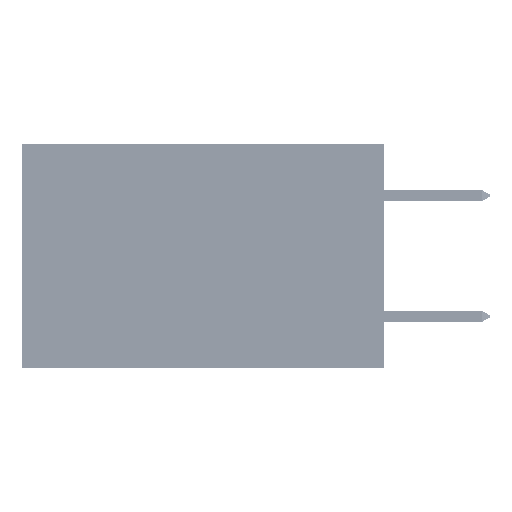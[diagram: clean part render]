
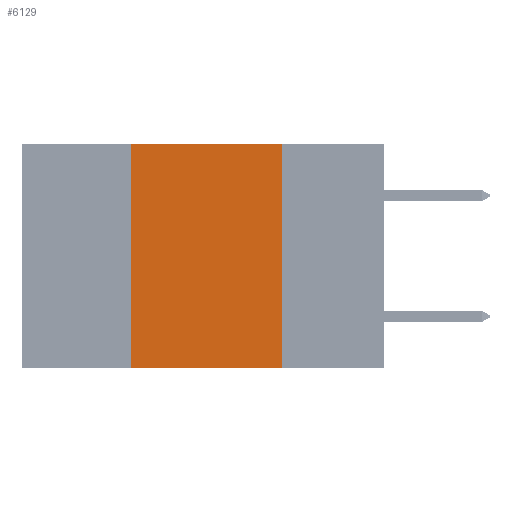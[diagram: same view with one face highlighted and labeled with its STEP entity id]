
A CAD part, left-side view. The second image highlights one B-rep face of the part: STEP entity #6129.
In plain terms, the highlighted planar face has unit normal (-1, 0, 0).
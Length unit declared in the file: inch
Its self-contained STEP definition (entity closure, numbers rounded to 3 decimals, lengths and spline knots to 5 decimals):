
#856 = EDGE_CURVE ( 'NONE', #33650, #27163, #22247, .T. ) ;
#1186 = VECTOR ( 'NONE', #45762, 39.37008 ) ;
#2209 = EDGE_CURVE ( 'NONE', #26394, #33452, #11056, .T. ) ;
#2856 = CARTESIAN_POINT ( 'NONE',  ( 0., 0.17, 0. ) ) ;
#3942 = EDGE_CURVE ( 'NONE', #26394, #33650, #14056, .T. ) ;
#6129 = ADVANCED_FACE ( 'NONE', ( #16277 ), #30497, .F. ) ;
#7517 = CARTESIAN_POINT ( 'NONE',  ( 0., 0.42, 0. ) ) ;
#9298 = DIRECTION ( 'NONE',  ( 0., 0., -1. ) ) ;
#10473 = DIRECTION ( 'NONE',  ( 0., 0., -1. ) ) ;
#10934 = CARTESIAN_POINT ( 'NONE',  ( 0., 0.42, -0.37 ) ) ;
#11056 = LINE ( 'NONE', #17357, #1186 ) ;
#11306 = ORIENTED_EDGE ( 'NONE', *, *, #2209, .T. ) ;
#12801 = DIRECTION ( 'NONE',  ( 1., 0., 0. ) ) ;
#13345 = CARTESIAN_POINT ( 'NONE',  ( 0., 0.17, -0.37 ) ) ;
#13594 = AXIS2_PLACEMENT_3D ( 'NONE', #44694, #12801, #9298 ) ;
#14056 = LINE ( 'NONE', #7517, #21716 ) ;
#15438 = VECTOR ( 'NONE', #33174, 39.37008 ) ;
#16277 = FACE_OUTER_BOUND ( 'NONE', #37872, .T. ) ;
#17357 = CARTESIAN_POINT ( 'NONE',  ( 0., 0.6, -0.37 ) ) ;
#19200 = CARTESIAN_POINT ( 'NONE',  ( 0., 0.6, 0. ) ) ;
#21716 = VECTOR ( 'NONE', #28941, 39.37008 ) ;
#22247 = LINE ( 'NONE', #19200, #15438 ) ;
#22979 = ORIENTED_EDGE ( 'NONE', *, *, #31067, .F. ) ;
#23288 = CARTESIAN_POINT ( 'NONE',  ( 0., 0.42, 0. ) ) ;
#26394 = VERTEX_POINT ( 'NONE', #10934 ) ;
#27163 = VERTEX_POINT ( 'NONE', #2856 ) ;
#27729 = VECTOR ( 'NONE', #10473, 39.37008 ) ;
#28852 = LINE ( 'NONE', #35614, #27729 ) ;
#28941 = DIRECTION ( 'NONE',  ( 0., 0., 1. ) ) ;
#30497 = PLANE ( 'NONE',  #13594 ) ;
#31067 = EDGE_CURVE ( 'NONE', #27163, #33452, #28852, .T. ) ;
#33174 = DIRECTION ( 'NONE',  ( 0., -1., 0. ) ) ;
#33452 = VERTEX_POINT ( 'NONE', #13345 ) ;
#33650 = VERTEX_POINT ( 'NONE', #23288 ) ;
#35614 = CARTESIAN_POINT ( 'NONE',  ( 0., 0.17, 0. ) ) ;
#37299 = ORIENTED_EDGE ( 'NONE', *, *, #3942, .F. ) ;
#37872 = EDGE_LOOP ( 'NONE', ( #22979, #42154, #37299, #11306 ) ) ;
#42154 = ORIENTED_EDGE ( 'NONE', *, *, #856, .F. ) ;
#44694 = CARTESIAN_POINT ( 'NONE',  ( 0., 0.6, 0. ) ) ;
#45762 = DIRECTION ( 'NONE',  ( 0., -1., 0. ) ) ;
